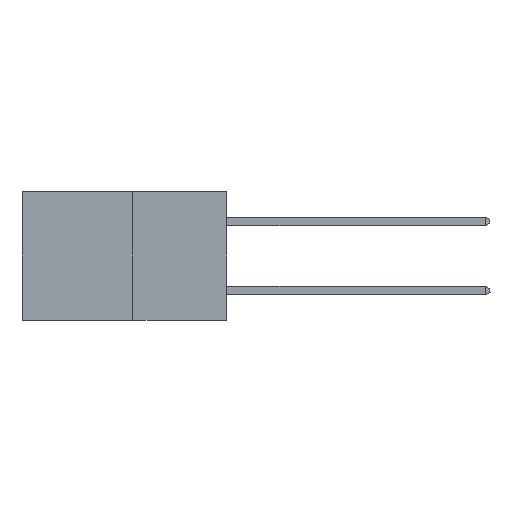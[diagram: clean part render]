
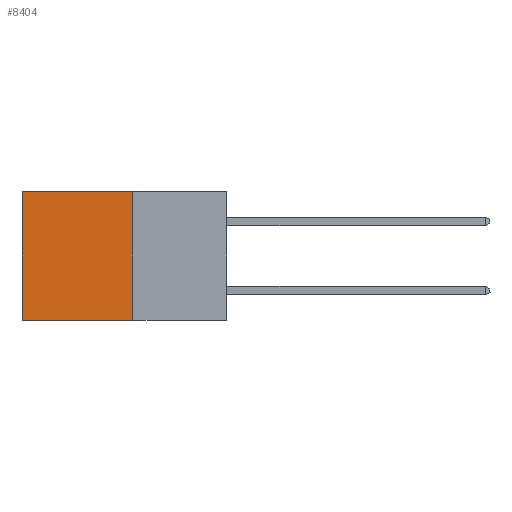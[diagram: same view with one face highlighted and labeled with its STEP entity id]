
A CAD part, left-side view. The second image highlights one B-rep face of the part: STEP entity #8404.
In plain terms, the highlighted planar face has unit normal (-1, 0, 0).
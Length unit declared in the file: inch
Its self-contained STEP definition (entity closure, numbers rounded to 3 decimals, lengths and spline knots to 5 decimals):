
#190 = ORIENTED_EDGE ( 'NONE', *, *, #2185, .T. ) ;
#713 = ORIENTED_EDGE ( 'NONE', *, *, #5334, .F. ) ;
#820 = DIRECTION ( 'NONE',  ( 0., 1., 0. ) ) ;
#1159 = CARTESIAN_POINT ( 'NONE',  ( 0.277, 0.59, -0.37 ) ) ;
#1269 = VECTOR ( 'NONE', #2019, 39.37008 ) ;
#1945 = EDGE_CURVE ( 'NONE', #7396, #6652, #5934, .T. ) ;
#2019 = DIRECTION ( 'NONE',  ( 0., 0., -1. ) ) ;
#2091 = DIRECTION ( 'NONE',  ( 0., 0., -1. ) ) ;
#2185 = EDGE_CURVE ( 'NONE', #6652, #6407, #2895, .T. ) ;
#2547 = CARTESIAN_POINT ( 'NONE',  ( 0.277, 0.27, 0. ) ) ;
#2895 = LINE ( 'NONE', #8175, #8545 ) ;
#3724 = DIRECTION ( 'NONE',  ( 0., 0., -1. ) ) ;
#3828 = CARTESIAN_POINT ( 'NONE',  ( 0.277, 0.27, -0.37 ) ) ;
#4496 = CARTESIAN_POINT ( 'NONE',  ( 0.277, 0.27, -0.37 ) ) ;
#5334 = EDGE_CURVE ( 'NONE', #9201, #6407, #7593, .T. ) ;
#5668 = ORIENTED_EDGE ( 'NONE', *, *, #5924, .F. ) ;
#5924 = EDGE_CURVE ( 'NONE', #7396, #9201, #7578, .T. ) ;
#5934 = LINE ( 'NONE', #9563, #9167 ) ;
#6253 = ORIENTED_EDGE ( 'NONE', *, *, #1945, .T. ) ;
#6407 = VERTEX_POINT ( 'NONE', #1159 ) ;
#6509 = CARTESIAN_POINT ( 'NONE',  ( 0.277, 0.27, -0.37 ) ) ;
#6639 = EDGE_LOOP ( 'NONE', ( #190, #713, #5668, #6253 ) ) ;
#6652 = VERTEX_POINT ( 'NONE', #8816 ) ;
#6904 = DIRECTION ( 'NONE',  ( 1., 0., 0. ) ) ;
#7061 = CARTESIAN_POINT ( 'NONE',  ( 0.277, 0.27, -0.37 ) ) ;
#7199 = AXIS2_PLACEMENT_3D ( 'NONE', #4496, #6904, #2091 ) ;
#7396 = VERTEX_POINT ( 'NONE', #2547 ) ;
#7578 = LINE ( 'NONE', #7061, #1269 ) ;
#7593 = LINE ( 'NONE', #6509, #9148 ) ;
#7749 = DIRECTION ( 'NONE',  ( 0., 1., 0. ) ) ;
#8117 = PLANE ( 'NONE',  #7199 ) ;
#8175 = CARTESIAN_POINT ( 'NONE',  ( 0.277, 0.59, -0.37 ) ) ;
#8404 = ADVANCED_FACE ( 'NONE', ( #8428 ), #8117, .F. ) ;
#8428 = FACE_OUTER_BOUND ( 'NONE', #6639, .T. ) ;
#8545 = VECTOR ( 'NONE', #3724, 39.37008 ) ;
#8816 = CARTESIAN_POINT ( 'NONE',  ( 0.277, 0.59, 0. ) ) ;
#9148 = VECTOR ( 'NONE', #7749, 39.37008 ) ;
#9167 = VECTOR ( 'NONE', #820, 39.37008 ) ;
#9201 = VERTEX_POINT ( 'NONE', #3828 ) ;
#9563 = CARTESIAN_POINT ( 'NONE',  ( 0.277, 0.27, 0. ) ) ;
